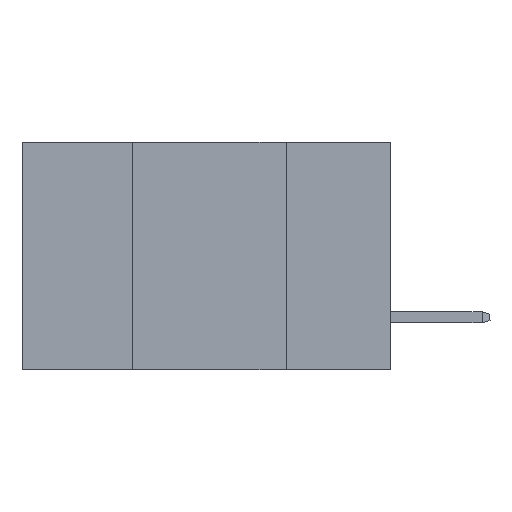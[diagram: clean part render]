
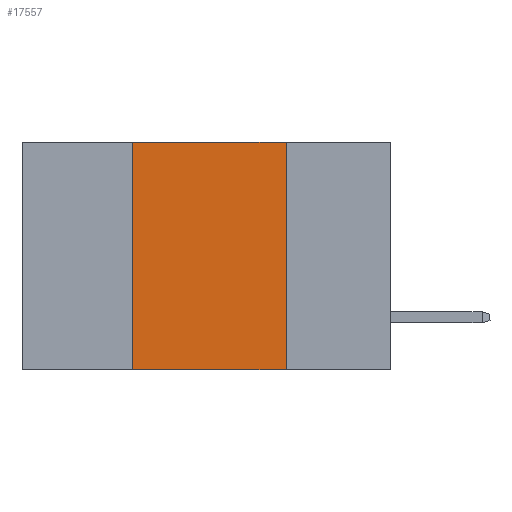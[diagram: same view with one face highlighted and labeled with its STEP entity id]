
A CAD part, left-side view. The second image highlights one B-rep face of the part: STEP entity #17557.
In plain terms, the highlighted planar face has unit normal (-1, 0, 0).
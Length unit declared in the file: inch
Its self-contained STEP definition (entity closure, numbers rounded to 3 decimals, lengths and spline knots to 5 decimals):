
#356 = DIRECTION ( 'NONE',  ( 0., 0., 1. ) ) ;
#1181 = ORIENTED_EDGE ( 'NONE', *, *, #7987, .F. ) ;
#1504 = LINE ( 'NONE', #9405, #10237 ) ;
#3800 = CARTESIAN_POINT ( 'NONE',  ( 0., 0.6, -0.37 ) ) ;
#4228 = DIRECTION ( 'NONE',  ( 0., -1., 0. ) ) ;
#4319 = CARTESIAN_POINT ( 'NONE',  ( 0., 0.42, -0.37 ) ) ;
#4574 = EDGE_CURVE ( 'NONE', #15785, #17120, #15292, .T. ) ;
#5314 = AXIS2_PLACEMENT_3D ( 'NONE', #16154, #19540, #9277 ) ;
#5581 = DIRECTION ( 'NONE',  ( 0., -1., 0. ) ) ;
#7042 = CARTESIAN_POINT ( 'NONE',  ( 0., 0.17, 0. ) ) ;
#7987 = EDGE_CURVE ( 'NONE', #11078, #11120, #1504, .T. ) ;
#9055 = VECTOR ( 'NONE', #19584, 39.37008 ) ;
#9277 = DIRECTION ( 'NONE',  ( 0., 0., -1. ) ) ;
#9405 = CARTESIAN_POINT ( 'NONE',  ( 0., 0.6, 0. ) ) ;
#10237 = VECTOR ( 'NONE', #4228, 39.37008 ) ;
#10310 = ORIENTED_EDGE ( 'NONE', *, *, #10774, .F. ) ;
#10635 = VECTOR ( 'NONE', #356, 39.37008 ) ;
#10774 = EDGE_CURVE ( 'NONE', #11120, #17120, #13652, .T. ) ;
#10787 = FACE_OUTER_BOUND ( 'NONE', #19427, .T. ) ;
#11040 = CARTESIAN_POINT ( 'NONE',  ( 0., 0.17, 0. ) ) ;
#11078 = VERTEX_POINT ( 'NONE', #22111 ) ;
#11120 = VERTEX_POINT ( 'NONE', #7042 ) ;
#11196 = LINE ( 'NONE', #21136, #10635 ) ;
#13652 = LINE ( 'NONE', #11040, #9055 ) ;
#14732 = VECTOR ( 'NONE', #5581, 39.37008 ) ;
#15292 = LINE ( 'NONE', #3800, #14732 ) ;
#15785 = VERTEX_POINT ( 'NONE', #4319 ) ;
#15801 = ORIENTED_EDGE ( 'NONE', *, *, #19993, .F. ) ;
#16082 = PLANE ( 'NONE',  #5314 ) ;
#16154 = CARTESIAN_POINT ( 'NONE',  ( 0., 0.6, 0. ) ) ;
#16667 = CARTESIAN_POINT ( 'NONE',  ( 0., 0.17, -0.37 ) ) ;
#17120 = VERTEX_POINT ( 'NONE', #16667 ) ;
#17557 = ADVANCED_FACE ( 'NONE', ( #10787 ), #16082, .F. ) ;
#19427 = EDGE_LOOP ( 'NONE', ( #10310, #1181, #15801, #20575 ) ) ;
#19540 = DIRECTION ( 'NONE',  ( 1., 0., 0. ) ) ;
#19584 = DIRECTION ( 'NONE',  ( 0., 0., -1. ) ) ;
#19993 = EDGE_CURVE ( 'NONE', #15785, #11078, #11196, .T. ) ;
#20575 = ORIENTED_EDGE ( 'NONE', *, *, #4574, .T. ) ;
#21136 = CARTESIAN_POINT ( 'NONE',  ( 0., 0.42, 0. ) ) ;
#22111 = CARTESIAN_POINT ( 'NONE',  ( 0., 0.42, 0. ) ) ;
